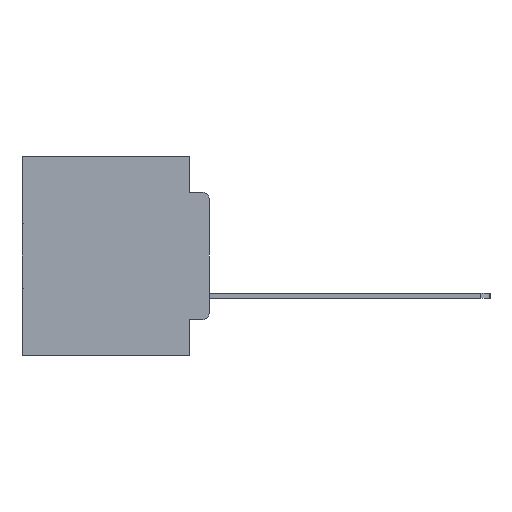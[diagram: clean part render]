
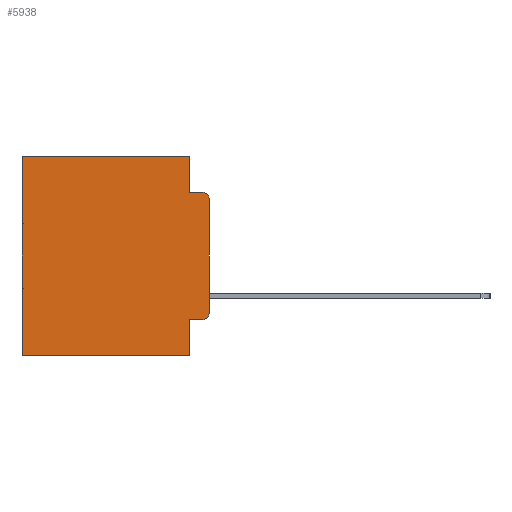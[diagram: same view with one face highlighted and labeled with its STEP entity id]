
A CAD part, left-side view. The second image highlights one B-rep face of the part: STEP entity #5938.
In plain terms, the highlighted planar face has unit normal (-1, 0, 0).
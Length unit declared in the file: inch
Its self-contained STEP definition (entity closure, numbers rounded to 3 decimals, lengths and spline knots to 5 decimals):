
#1425 = VECTOR ( 'NONE', #11672, 39.37008 ) ;
#2060 = EDGE_CURVE ( 'NONE', #12956, #30396, #5543, .T. ) ;
#2313 = ORIENTED_EDGE ( 'NONE', *, *, #31496, .T. ) ;
#2513 = EDGE_CURVE ( 'NONE', #24956, #13496, #30471, .T. ) ;
#2752 = CARTESIAN_POINT ( 'NONE',  ( 0.298, 0.051, -0.0885 ) ) ;
#3287 = CARTESIAN_POINT ( 'NONE',  ( 0.298, 0.051, -0.0885 ) ) ;
#3526 = ORIENTED_EDGE ( 'NONE', *, *, #18065, .T. ) ;
#3572 = AXIS2_PLACEMENT_3D ( 'NONE', #4347, #9507, #26940 ) ;
#3646 = VERTEX_POINT ( 'NONE', #3287 ) ;
#4347 = CARTESIAN_POINT ( 'NONE',  ( 0.298, 0., 0. ) ) ;
#4573 = DIRECTION ( 'NONE',  ( 0., 0., -1. ) ) ;
#4710 = ORIENTED_EDGE ( 'NONE', *, *, #8986, .F. ) ;
#5203 = DIRECTION ( 'NONE',  ( 0., 0., -1. ) ) ;
#5421 = VERTEX_POINT ( 'NONE', #12711 ) ;
#5543 = CIRCLE ( 'NONE', #18596, 0.02 ) ;
#5546 = VECTOR ( 'NONE', #4573, 39.37008 ) ;
#5795 = VERTEX_POINT ( 'NONE', #26408 ) ;
#5938 = ADVANCED_FACE ( 'NONE', ( #7336 ), #24364, .F. ) ;
#6063 = DIRECTION ( 'NONE',  ( -1., 0., 0. ) ) ;
#6129 = LINE ( 'NONE', #10266, #7733 ) ;
#7336 = FACE_OUTER_BOUND ( 'NONE', #18098, .T. ) ;
#7733 = VECTOR ( 'NONE', #5203, 39.37008 ) ;
#8469 = VECTOR ( 'NONE', #24017, 39.37008 ) ;
#8986 = EDGE_CURVE ( 'NONE', #12956, #12643, #26312, .T. ) ;
#9159 = LINE ( 'NONE', #22289, #29003 ) ;
#9507 = DIRECTION ( 'NONE',  ( 1., 0., 0. ) ) ;
#10266 = CARTESIAN_POINT ( 'NONE',  ( 0.298, 0.051, 0. ) ) ;
#11370 = VERTEX_POINT ( 'NONE', #19261 ) ;
#11672 = DIRECTION ( 'NONE',  ( 0., 0., -1. ) ) ;
#11680 = VECTOR ( 'NONE', #20001, 39.37008 ) ;
#11691 = CARTESIAN_POINT ( 'NONE',  ( 0.298, 0.02, -0.0885 ) ) ;
#11705 = CARTESIAN_POINT ( 'NONE',  ( 0.298, 0.02, -0.3915 ) ) ;
#12643 = VERTEX_POINT ( 'NONE', #18593 ) ;
#12711 = CARTESIAN_POINT ( 'NONE',  ( 0.298, 0.02, -0.4115 ) ) ;
#12956 = VERTEX_POINT ( 'NONE', #27191 ) ;
#13496 = VERTEX_POINT ( 'NONE', #31720 ) ;
#14115 = CARTESIAN_POINT ( 'NONE',  ( 0.298, 0., 0. ) ) ;
#14292 = DIRECTION ( 'NONE',  ( 0., 0., -1. ) ) ;
#15255 = LINE ( 'NONE', #14115, #8469 ) ;
#15458 = ORIENTED_EDGE ( 'NONE', *, *, #27953, .F. ) ;
#15615 = AXIS2_PLACEMENT_3D ( 'NONE', #11705, #29014, #14292 ) ;
#15946 = VERTEX_POINT ( 'NONE', #22922 ) ;
#16160 = ORIENTED_EDGE ( 'NONE', *, *, #2513, .F. ) ;
#17212 = VECTOR ( 'NONE', #22968, 39.37008 ) ;
#17503 = CARTESIAN_POINT ( 'NONE',  ( 0.298, 0.473, 0. ) ) ;
#18065 = EDGE_CURVE ( 'NONE', #5421, #12643, #19039, .T. ) ;
#18098 = EDGE_LOOP ( 'NONE', ( #4710, #30469, #22446, #15458, #2313, #26742, #16160, #19919, #31358, #3526 ) ) ;
#18192 = VECTOR ( 'NONE', #25404, 39.37008 ) ;
#18593 = CARTESIAN_POINT ( 'NONE',  ( 0.298, 0., -0.3915 ) ) ;
#18596 = AXIS2_PLACEMENT_3D ( 'NONE', #21135, #6063, #23611 ) ;
#19039 = CIRCLE ( 'NONE', #15615, 0.02 ) ;
#19261 = CARTESIAN_POINT ( 'NONE',  ( 0.298, 0.051, -0.4115 ) ) ;
#19705 = DIRECTION ( 'NONE',  ( 0., -1., 0. ) ) ;
#19919 = ORIENTED_EDGE ( 'NONE', *, *, #23031, .F. ) ;
#20001 = DIRECTION ( 'NONE',  ( 0., 0., -1. ) ) ;
#21135 = CARTESIAN_POINT ( 'NONE',  ( 0.298, 0.02, -0.1085 ) ) ;
#21364 = EDGE_CURVE ( 'NONE', #11370, #5421, #9159, .T. ) ;
#21590 = CARTESIAN_POINT ( 'NONE',  ( 0.298, 0.051, 0. ) ) ;
#21657 = LINE ( 'NONE', #21590, #1425 ) ;
#22289 = CARTESIAN_POINT ( 'NONE',  ( 0.298, 0.051, -0.4115 ) ) ;
#22446 = ORIENTED_EDGE ( 'NONE', *, *, #31208, .F. ) ;
#22922 = CARTESIAN_POINT ( 'NONE',  ( 0.298, 0.051, 0. ) ) ;
#22968 = DIRECTION ( 'NONE',  ( 0., -1., 0. ) ) ;
#23031 = EDGE_CURVE ( 'NONE', #11370, #24956, #6129, .T. ) ;
#23611 = DIRECTION ( 'NONE',  ( 0., 0., -1. ) ) ;
#23628 = CARTESIAN_POINT ( 'NONE',  ( 0.298, 0.051, -0.5 ) ) ;
#24017 = DIRECTION ( 'NONE',  ( 0., 1., 0. ) ) ;
#24364 = PLANE ( 'NONE',  #3572 ) ;
#24532 = LINE ( 'NONE', #2752, #17212 ) ;
#24663 = EDGE_CURVE ( 'NONE', #5795, #13496, #31376, .T. ) ;
#24956 = VERTEX_POINT ( 'NONE', #23628 ) ;
#25404 = DIRECTION ( 'NONE',  ( 0., 1., 0. ) ) ;
#26312 = LINE ( 'NONE', #27032, #5546 ) ;
#26408 = CARTESIAN_POINT ( 'NONE',  ( 0.298, 0.473, 0. ) ) ;
#26742 = ORIENTED_EDGE ( 'NONE', *, *, #24663, .T. ) ;
#26940 = DIRECTION ( 'NONE',  ( 0., 0., -1. ) ) ;
#27032 = CARTESIAN_POINT ( 'NONE',  ( 0.298, 0., 0. ) ) ;
#27191 = CARTESIAN_POINT ( 'NONE',  ( 0.298, 0., -0.1085 ) ) ;
#27953 = EDGE_CURVE ( 'NONE', #15946, #3646, #21657, .T. ) ;
#29003 = VECTOR ( 'NONE', #19705, 39.37008 ) ;
#29014 = DIRECTION ( 'NONE',  ( -1., 0., 0. ) ) ;
#30317 = CARTESIAN_POINT ( 'NONE',  ( 0.298, 0., -0.5 ) ) ;
#30396 = VERTEX_POINT ( 'NONE', #11691 ) ;
#30469 = ORIENTED_EDGE ( 'NONE', *, *, #2060, .T. ) ;
#30471 = LINE ( 'NONE', #30317, #18192 ) ;
#31208 = EDGE_CURVE ( 'NONE', #3646, #30396, #24532, .T. ) ;
#31358 = ORIENTED_EDGE ( 'NONE', *, *, #21364, .T. ) ;
#31376 = LINE ( 'NONE', #17503, #11680 ) ;
#31496 = EDGE_CURVE ( 'NONE', #15946, #5795, #15255, .T. ) ;
#31720 = CARTESIAN_POINT ( 'NONE',  ( 0.298, 0.473, -0.5 ) ) ;
